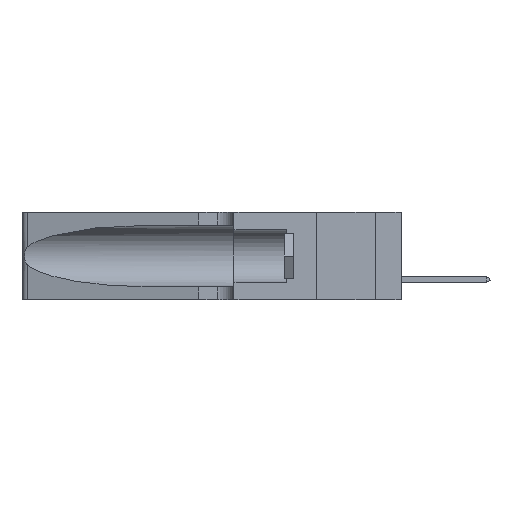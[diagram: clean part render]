
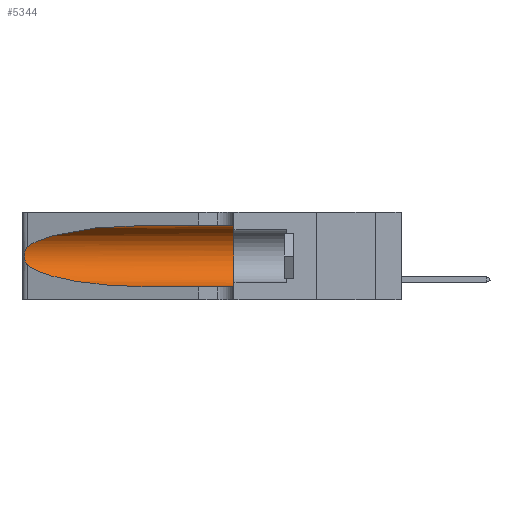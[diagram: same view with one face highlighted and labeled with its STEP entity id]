
A CAD part, left-side view. The second image highlights one B-rep face of the part: STEP entity #5344.
In plain terms, the highlighted cylindrical face has radius 3.308 mm (diameter 6.617 mm), a partial arc.
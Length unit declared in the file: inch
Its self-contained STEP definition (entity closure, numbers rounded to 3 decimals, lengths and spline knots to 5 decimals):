
#630 = CARTESIAN_POINT ( 'NONE',  ( 0.25487, 1.22718, 0.22369 ) ) ;
#722 = CARTESIAN_POINT ( 'NONE',  ( 0.25639, 1.23186, 0.15144 ) ) ;
#1498 = EDGE_CURVE ( 'NONE', #9878, #12883, #22788, .T. ) ;
#2052 = EDGE_CURVE ( 'NONE', #9878, #21538, #21624, .T. ) ;
#2401 = CARTESIAN_POINT ( 'NONE',  ( 0.25639, 1.23184, 0.21858 ) ) ;
#2990 = FACE_OUTER_BOUND ( 'NONE', #13513, .T. ) ;
#3007 = CARTESIAN_POINT ( 'NONE',  ( 0.1305, 1.61858, 0.05475 ) ) ;
#3152 = CARTESIAN_POINT ( 'NONE',  ( 0.1305, 0.35, 0.31525 ) ) ;
#4179 = CARTESIAN_POINT ( 'NONE',  ( 0.18966, 0.96281, 0.31525 ) ) ;
#4185 = CARTESIAN_POINT ( 'NONE',  ( 0.1305, 0.35, 0.185 ) ) ;
#4508 = DIRECTION ( 'NONE',  ( 0., -1., 0. ) ) ;
#4587 = ORIENTED_EDGE ( 'NONE', *, *, #1498, .F. ) ;
#5209 = ORIENTED_EDGE ( 'NONE', *, *, #20288, .T. ) ;
#5344 = ADVANCED_FACE ( 'NONE', ( #2990 ), #14842, .F. ) ;
#5505 = ORIENTED_EDGE ( 'NONE', *, *, #21631, .T. ) ;
#5655 = CARTESIAN_POINT ( 'NONE',  ( 0.25487, 1.22718, 0.22369 ) ) ;
#5901 = ORIENTED_EDGE ( 'NONE', *, *, #2052, .T. ) ;
#5954 = VECTOR ( 'NONE', #8782, 39.37008 ) ;
#5969 = CARTESIAN_POINT ( 'NONE',  ( 0.26018, 1.23835, 0.19895 ) ) ;
#5973 = DIRECTION ( 'NONE',  ( 0., -1., 0. ) ) ;
#6014 = VERTEX_POINT ( 'NONE', #22690 ) ;
#6151 = CARTESIAN_POINT ( 'NONE',  ( 0.1305, 1.61858, 0.31525 ) ) ;
#6618 = ORIENTED_EDGE ( 'NONE', *, *, #13828, .T. ) ;
#6811 = EDGE_CURVE ( 'NONE', #12883, #14127, #11223, .T. ) ;
#7665 = CARTESIAN_POINT ( 'NONE',  ( 0.25789, 1.23486, 0.15765 ) ) ;
#8782 = DIRECTION ( 'NONE',  ( 0., -1., 0. ) ) ;
#9352 = CARTESIAN_POINT ( 'NONE',  ( 0.1305, 0.72297, 0.05475 ) ) ;
#9428 = CARTESIAN_POINT ( 'NONE',  ( 0.25856, 1.23593, 0.16098 ) ) ;
#9505 = CARTESIAN_POINT ( 'NONE',  ( 0.25487, 1.22718, 0.22369 ) ) ;
#9659 = CARTESIAN_POINT ( 'NONE',  ( 0.25854, 1.2359, 0.20912 ) ) ;
#9878 = VERTEX_POINT ( 'NONE', #12767 ) ;
#10503 = B_SPLINE_CURVE_WITH_KNOTS ( 'NONE', 3,
 ( #9505, #20189, #2401, #16736, #9659, #5969, #16811, #11299, #18213, #9428, #7665, #722, #21738, #13072 ),
 .UNSPECIFIED., .F., .F.,
 ( 4, 2, 2, 2, 2, 2, 4 ),
 ( 0., 0.00027, 0.00053, 0.00107, 0.0016, 0.00187, 0.00214 ),
 .UNSPECIFIED. ) ;
#11065 = CARTESIAN_POINT ( 'NONE',  ( 0.25487, 1.22718, 0.14631 ) ) ;
#11202 = CARTESIAN_POINT ( 'NONE',  ( 0.2373, 1.15595, 0.28018 ) ) ;
#11223 = CIRCLE ( 'NONE', #17356, 0.13025 ) ;
#11299 = CARTESIAN_POINT ( 'NONE',  ( 0.26075, 1.23896, 0.178 ) ) ;
#12740 = DIRECTION ( 'NONE',  ( 0., 0., 1. ) ) ;
#12752 =( BOUNDED_CURVE ( )  B_SPLINE_CURVE ( 3, ( #11065, #13073, #18371, #9352 ),
 .UNSPECIFIED., .F., .F. ) 
 B_SPLINE_CURVE_WITH_KNOTS ( ( 4, 4 ),
 ( 3.44316, 4.71239 ),
 .UNSPECIFIED. ) 
 CURVE ( )  GEOMETRIC_REPRESENTATION_ITEM ( )  RATIONAL_B_SPLINE_CURVE ( ( 1., 0.87, 0.87, 1. ) ) 
 REPRESENTATION_ITEM ( '' )  );
#12767 = CARTESIAN_POINT ( 'NONE',  ( 0.1305, 0.72297, 0.31525 ) ) ;
#12883 = VERTEX_POINT ( 'NONE', #3152 ) ;
#13072 = CARTESIAN_POINT ( 'NONE',  ( 0.25487, 1.22718, 0.14631 ) ) ;
#13073 = CARTESIAN_POINT ( 'NONE',  ( 0.2373, 1.15595, 0.08982 ) ) ;
#13210 = CARTESIAN_POINT ( 'NONE',  ( 0.1305, 0.72297, 0.31525 ) ) ;
#13513 = EDGE_LOOP ( 'NONE', ( #5901, #5505, #6618, #5209, #22074, #4587 ) ) ;
#13828 = EDGE_CURVE ( 'NONE', #6014, #16046, #12752, .T. ) ;
#13941 = CARTESIAN_POINT ( 'NONE',  ( 0.1305, 0.72297, 0.05475 ) ) ;
#14127 = VERTEX_POINT ( 'NONE', #17196 ) ;
#14596 = DIRECTION ( 'NONE',  ( 0., 1., 0. ) ) ;
#14842 = CYLINDRICAL_SURFACE ( 'NONE', #19115, 0.13025 ) ;
#16046 = VERTEX_POINT ( 'NONE', #13941 ) ;
#16413 = LINE ( 'NONE', #3007, #5954 ) ;
#16736 = CARTESIAN_POINT ( 'NONE',  ( 0.25787, 1.23484, 0.2124 ) ) ;
#16811 = CARTESIAN_POINT ( 'NONE',  ( 0.26075, 1.23896, 0.19203 ) ) ;
#17196 = CARTESIAN_POINT ( 'NONE',  ( 0.1305, 0.35, 0.05475 ) ) ;
#17356 = AXIS2_PLACEMENT_3D ( 'NONE', #4185, #14596, #12740 ) ;
#18113 = VECTOR ( 'NONE', #4508, 39.37008 ) ;
#18213 = CARTESIAN_POINT ( 'NONE',  ( 0.26017, 1.23833, 0.17102 ) ) ;
#18217 = DIRECTION ( 'NONE',  ( 0., 0., -1. ) ) ;
#18371 = CARTESIAN_POINT ( 'NONE',  ( 0.18966, 0.96281, 0.05475 ) ) ;
#19115 = AXIS2_PLACEMENT_3D ( 'NONE', #21585, #5973, #18217 ) ;
#20189 = CARTESIAN_POINT ( 'NONE',  ( 0.25555, 1.22994, 0.2215 ) ) ;
#20288 = EDGE_CURVE ( 'NONE', #16046, #14127, #16413, .T. ) ;
#21538 = VERTEX_POINT ( 'NONE', #5655 ) ;
#21585 = CARTESIAN_POINT ( 'NONE',  ( 0.1305, 1.61858, 0.185 ) ) ;
#21624 =( BOUNDED_CURVE ( )  B_SPLINE_CURVE ( 3, ( #13210, #4179, #11202, #630 ),
 .UNSPECIFIED., .F., .F. ) 
 B_SPLINE_CURVE_WITH_KNOTS ( ( 4, 4 ),
 ( 1.5708, 2.84003 ),
 .UNSPECIFIED. ) 
 CURVE ( )  GEOMETRIC_REPRESENTATION_ITEM ( )  RATIONAL_B_SPLINE_CURVE ( ( 1., 0.87, 0.87, 1. ) ) 
 REPRESENTATION_ITEM ( '' )  );
#21631 = EDGE_CURVE ( 'NONE', #21538, #6014, #10503, .T. ) ;
#21738 = CARTESIAN_POINT ( 'NONE',  ( 0.25555, 1.22993, 0.14849 ) ) ;
#22074 = ORIENTED_EDGE ( 'NONE', *, *, #6811, .F. ) ;
#22690 = CARTESIAN_POINT ( 'NONE',  ( 0.25487, 1.22718, 0.14631 ) ) ;
#22788 = LINE ( 'NONE', #6151, #18113 ) ;
